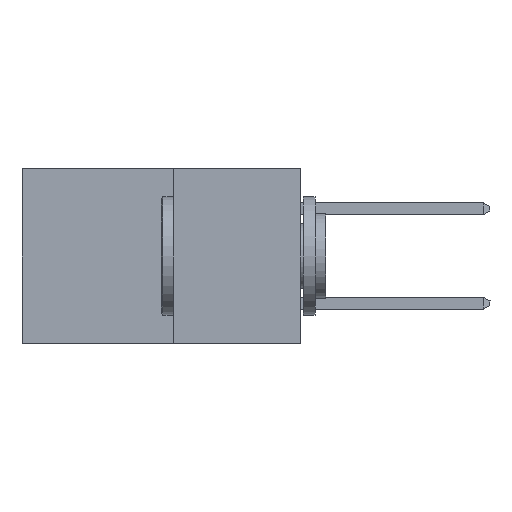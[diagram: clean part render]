
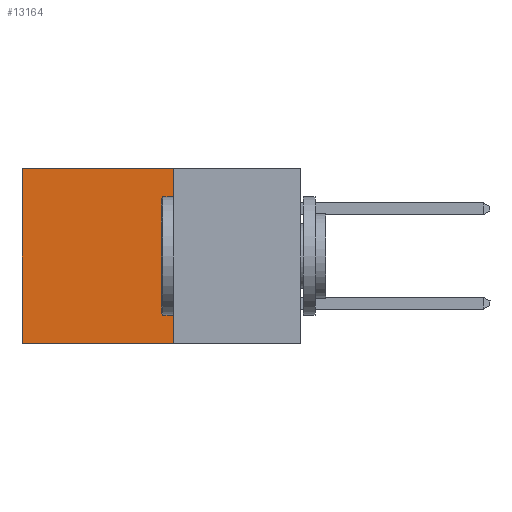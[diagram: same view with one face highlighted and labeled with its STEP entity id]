
A CAD part, left-side view. The second image highlights one B-rep face of the part: STEP entity #13164.
In plain terms, the highlighted planar face has unit normal (-1, 0, 0).
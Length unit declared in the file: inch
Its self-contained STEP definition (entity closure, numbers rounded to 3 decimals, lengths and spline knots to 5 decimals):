
#4543 = DIRECTION ( 'NONE',  ( 1., 0., 0. ) ) ;
#4560 = ORIENTED_EDGE ( 'NONE', *, *, #23617, .T. ) ;
#6059 = EDGE_CURVE ( 'NONE', #29686, #28866, #20840, .T. ) ;
#7833 = FACE_OUTER_BOUND ( 'NONE', #23335, .T. ) ;
#8266 = CARTESIAN_POINT ( 'NONE',  ( 0.277, 0.27, 0. ) ) ;
#9364 = DIRECTION ( 'NONE',  ( 0., 0., -1. ) ) ;
#9519 = CARTESIAN_POINT ( 'NONE',  ( 0.277, 0.27, -0.37 ) ) ;
#10163 = ORIENTED_EDGE ( 'NONE', *, *, #6059, .F. ) ;
#10882 = VERTEX_POINT ( 'NONE', #33255 ) ;
#11750 = AXIS2_PLACEMENT_3D ( 'NONE', #15167, #4543, #23156 ) ;
#13164 = ADVANCED_FACE ( 'NONE', ( #7833 ), #17742, .F. ) ;
#13841 = VECTOR ( 'NONE', #13844, 39.37008 ) ;
#13844 = DIRECTION ( 'NONE',  ( 0., 1., 0. ) ) ;
#14155 = ORIENTED_EDGE ( 'NONE', *, *, #19148, .F. ) ;
#15167 = CARTESIAN_POINT ( 'NONE',  ( 0.277, 0.27, -0.37 ) ) ;
#15713 = VERTEX_POINT ( 'NONE', #25193 ) ;
#17742 = PLANE ( 'NONE',  #11750 ) ;
#19056 = CARTESIAN_POINT ( 'NONE',  ( 0.277, 0.27, -0.37 ) ) ;
#19148 = EDGE_CURVE ( 'NONE', #28866, #15713, #30182, .T. ) ;
#20001 = VECTOR ( 'NONE', #9364, 39.37008 ) ;
#20145 = VECTOR ( 'NONE', #32218, 39.37008 ) ;
#20840 = LINE ( 'NONE', #9519, #20001 ) ;
#20993 = LINE ( 'NONE', #21640, #20145 ) ;
#21409 = ORIENTED_EDGE ( 'NONE', *, *, #22224, .T. ) ;
#21640 = CARTESIAN_POINT ( 'NONE',  ( 0.277, 0.59, -0.37 ) ) ;
#22224 = EDGE_CURVE ( 'NONE', #10882, #15713, #20993, .T. ) ;
#23156 = DIRECTION ( 'NONE',  ( 0., 0., -1. ) ) ;
#23335 = EDGE_LOOP ( 'NONE', ( #21409, #14155, #10163, #4560 ) ) ;
#23617 = EDGE_CURVE ( 'NONE', #29686, #10882, #28740, .T. ) ;
#25193 = CARTESIAN_POINT ( 'NONE',  ( 0.277, 0.59, -0.37 ) ) ;
#28162 = DIRECTION ( 'NONE',  ( 0., 1., 0. ) ) ;
#28554 = VECTOR ( 'NONE', #28162, 39.37008 ) ;
#28740 = LINE ( 'NONE', #8266, #13841 ) ;
#28866 = VERTEX_POINT ( 'NONE', #19056 ) ;
#29686 = VERTEX_POINT ( 'NONE', #30048 ) ;
#30048 = CARTESIAN_POINT ( 'NONE',  ( 0.277, 0.27, 0. ) ) ;
#30182 = LINE ( 'NONE', #30798, #28554 ) ;
#30798 = CARTESIAN_POINT ( 'NONE',  ( 0.277, 0.27, -0.37 ) ) ;
#32218 = DIRECTION ( 'NONE',  ( 0., 0., -1. ) ) ;
#33255 = CARTESIAN_POINT ( 'NONE',  ( 0.277, 0.59, 0. ) ) ;
